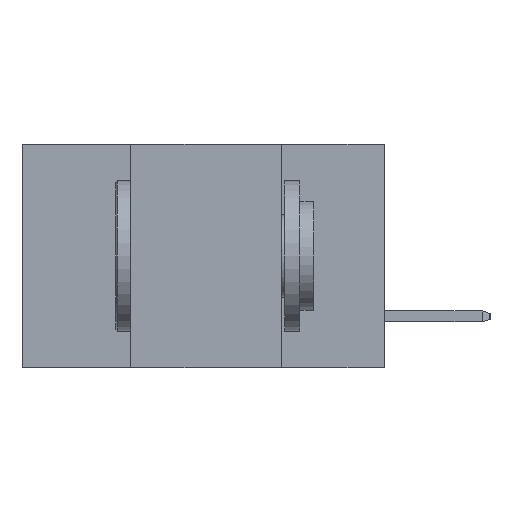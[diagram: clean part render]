
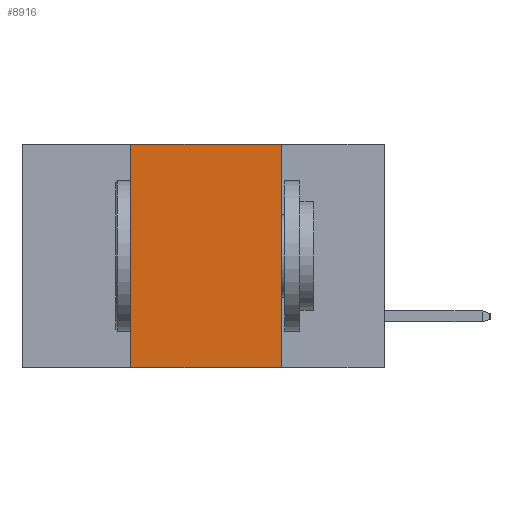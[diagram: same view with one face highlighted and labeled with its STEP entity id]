
A CAD part, left-side view. The second image highlights one B-rep face of the part: STEP entity #8916.
In plain terms, the highlighted planar face has unit normal (-1, 0, 0).
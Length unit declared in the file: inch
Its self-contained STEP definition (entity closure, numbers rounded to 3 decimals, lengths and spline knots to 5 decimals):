
#356 = VECTOR ( 'NONE', #9504, 39.37008 ) ;
#835 = EDGE_CURVE ( 'NONE', #1395, #2243, #8468, .T. ) ;
#1395 = VERTEX_POINT ( 'NONE', #6820 ) ;
#1446 = CARTESIAN_POINT ( 'NONE',  ( 0., 0.6, -0.37 ) ) ;
#1452 = CARTESIAN_POINT ( 'NONE',  ( 0., 0.6, 0. ) ) ;
#1532 = EDGE_CURVE ( 'NONE', #2243, #8143, #10689, .T. ) ;
#1594 = FACE_OUTER_BOUND ( 'NONE', #1683, .T. ) ;
#1683 = EDGE_LOOP ( 'NONE', ( #9805, #7713, #2674, #6108 ) ) ;
#2076 = LINE ( 'NONE', #3604, #7095 ) ;
#2243 = VERTEX_POINT ( 'NONE', #10006 ) ;
#2525 = CARTESIAN_POINT ( 'NONE',  ( 0., 0.17, -0.37 ) ) ;
#2674 = ORIENTED_EDGE ( 'NONE', *, *, #8037, .F. ) ;
#3565 = DIRECTION ( 'NONE',  ( 0., 0., 1. ) ) ;
#3604 = CARTESIAN_POINT ( 'NONE',  ( 0., 0.42, -0.37 ) ) ;
#3648 = CARTESIAN_POINT ( 'NONE',  ( 0., 0.42, -0.37 ) ) ;
#5657 = LINE ( 'NONE', #1446, #356 ) ;
#5727 = EDGE_CURVE ( 'NONE', #6488, #8143, #5657, .T. ) ;
#5907 = VECTOR ( 'NONE', #11603, 39.37008 ) ;
#6108 = ORIENTED_EDGE ( 'NONE', *, *, #5727, .T. ) ;
#6488 = VERTEX_POINT ( 'NONE', #3648 ) ;
#6563 = VECTOR ( 'NONE', #6774, 39.37008 ) ;
#6762 = CARTESIAN_POINT ( 'NONE',  ( 0., 0.17, -0.37 ) ) ;
#6774 = DIRECTION ( 'NONE',  ( 0., 0., -1. ) ) ;
#6820 = CARTESIAN_POINT ( 'NONE',  ( 0., 0.42, 0. ) ) ;
#7095 = VECTOR ( 'NONE', #3565, 39.37008 ) ;
#7713 = ORIENTED_EDGE ( 'NONE', *, *, #835, .F. ) ;
#7720 = DIRECTION ( 'NONE',  ( 0., 0., -1. ) ) ;
#7967 = DIRECTION ( 'NONE',  ( 1., 0., 0. ) ) ;
#8037 = EDGE_CURVE ( 'NONE', #6488, #1395, #2076, .T. ) ;
#8143 = VERTEX_POINT ( 'NONE', #2525 ) ;
#8187 = CARTESIAN_POINT ( 'NONE',  ( 0., 0.6, 0. ) ) ;
#8436 = PLANE ( 'NONE',  #9597 ) ;
#8468 = LINE ( 'NONE', #1452, #5907 ) ;
#8916 = ADVANCED_FACE ( 'NONE', ( #1594 ), #8436, .F. ) ;
#9504 = DIRECTION ( 'NONE',  ( 0., -1., 0. ) ) ;
#9597 = AXIS2_PLACEMENT_3D ( 'NONE', #8187, #7967, #7720 ) ;
#9805 = ORIENTED_EDGE ( 'NONE', *, *, #1532, .F. ) ;
#10006 = CARTESIAN_POINT ( 'NONE',  ( 0., 0.17, 0. ) ) ;
#10689 = LINE ( 'NONE', #6762, #6563 ) ;
#11603 = DIRECTION ( 'NONE',  ( 0., -1., 0. ) ) ;
